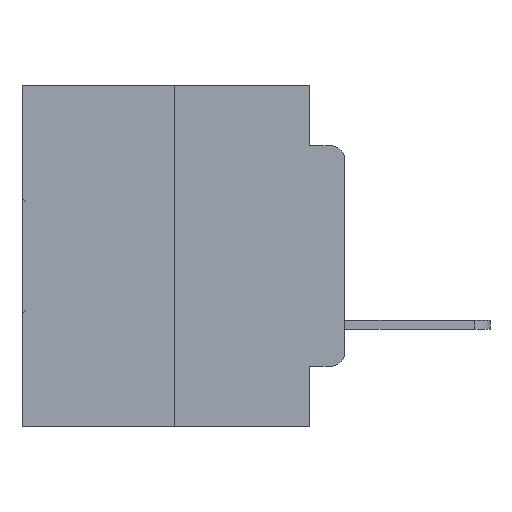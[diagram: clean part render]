
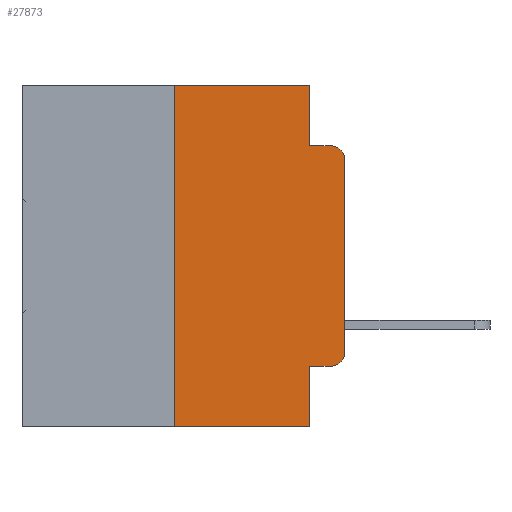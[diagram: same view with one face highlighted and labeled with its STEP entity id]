
A CAD part, left-side view. The second image highlights one B-rep face of the part: STEP entity #27873.
In plain terms, the highlighted planar face has unit normal (-1, 0, 0).
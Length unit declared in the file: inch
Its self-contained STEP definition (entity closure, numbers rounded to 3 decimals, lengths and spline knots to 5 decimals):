
#221 = EDGE_CURVE ( 'NONE', #346, #28090, #28840, .T. ) ;
#346 = VERTEX_POINT ( 'NONE', #8007 ) ;
#609 = LINE ( 'NONE', #29104, #14653 ) ;
#1253 = LINE ( 'NONE', #19078, #19991 ) ;
#1327 = EDGE_CURVE ( 'NONE', #11080, #346, #2122, .T. ) ;
#1549 = LINE ( 'NONE', #21572, #26983 ) ;
#1597 = VERTEX_POINT ( 'NONE', #19751 ) ;
#2122 = LINE ( 'NONE', #22585, #26089 ) ;
#2338 = CARTESIAN_POINT ( 'NONE',  ( 0., 0.02, -0.1085 ) ) ;
#3059 = ORIENTED_EDGE ( 'NONE', *, *, #221, .T. ) ;
#4509 = DIRECTION ( 'NONE',  ( 0., 0., -1. ) ) ;
#4846 = CARTESIAN_POINT ( 'NONE',  ( 0., 0.051, 0. ) ) ;
#5404 = CIRCLE ( 'NONE', #16463, 0.02 ) ;
#5990 = EDGE_CURVE ( 'NONE', #29400, #18457, #9635, .T. ) ;
#6635 = ORIENTED_EDGE ( 'NONE', *, *, #21454, .F. ) ;
#6990 = VERTEX_POINT ( 'NONE', #26063 ) ;
#7189 = DIRECTION ( 'NONE',  ( 0., 0., -1. ) ) ;
#7617 = LINE ( 'NONE', #24339, #30038 ) ;
#7746 = VERTEX_POINT ( 'NONE', #29175 ) ;
#7971 = DIRECTION ( 'NONE',  ( 0., -1., 0. ) ) ;
#7972 = CARTESIAN_POINT ( 'NONE',  ( 0., 0., -0.3915 ) ) ;
#8007 = CARTESIAN_POINT ( 'NONE',  ( 0., 0., -0.1085 ) ) ;
#8150 = EDGE_CURVE ( 'NONE', #6990, #7746, #1549, .T. ) ;
#8994 = VERTEX_POINT ( 'NONE', #11592 ) ;
#9467 = VERTEX_POINT ( 'NONE', #27816 ) ;
#9635 = LINE ( 'NONE', #15141, #26794 ) ;
#9763 = DIRECTION ( 'NONE',  ( 0., -1., 0. ) ) ;
#10082 = AXIS2_PLACEMENT_3D ( 'NONE', #27970, #18958, #4509 ) ;
#11080 = VERTEX_POINT ( 'NONE', #7972 ) ;
#11263 = ORIENTED_EDGE ( 'NONE', *, *, #1327, .T. ) ;
#11592 = CARTESIAN_POINT ( 'NONE',  ( 0., 0.051, -0.5 ) ) ;
#12137 = FACE_OUTER_BOUND ( 'NONE', #29045, .T. ) ;
#12693 = DIRECTION ( 'NONE',  ( 0., -1., 0. ) ) ;
#12794 = ORIENTED_EDGE ( 'NONE', *, *, #18736, .F. ) ;
#13134 = DIRECTION ( 'NONE',  ( 0., 0., -1. ) ) ;
#13972 = EDGE_CURVE ( 'NONE', #9467, #8994, #1253, .T. ) ;
#14167 = CARTESIAN_POINT ( 'NONE',  ( 0., 0.02, -0.3915 ) ) ;
#14268 = PLANE ( 'NONE',  #10082 ) ;
#14630 = EDGE_CURVE ( 'NONE', #1597, #28090, #7617, .T. ) ;
#14653 = VECTOR ( 'NONE', #13134, 39.37008 ) ;
#15141 = CARTESIAN_POINT ( 'NONE',  ( 0., 0.473, 0. ) ) ;
#15243 = LINE ( 'NONE', #19110, #20732 ) ;
#16463 = AXIS2_PLACEMENT_3D ( 'NONE', #14167, #30028, #16508 ) ;
#16508 = DIRECTION ( 'NONE',  ( 0., 0., -1. ) ) ;
#16810 = ORIENTED_EDGE ( 'NONE', *, *, #5990, .F. ) ;
#18341 = EDGE_CURVE ( 'NONE', #7746, #11080, #5404, .T. ) ;
#18457 = VERTEX_POINT ( 'NONE', #4846 ) ;
#18736 = EDGE_CURVE ( 'NONE', #18457, #1597, #15243, .T. ) ;
#18958 = DIRECTION ( 'NONE',  ( 1., 0., 0. ) ) ;
#19078 = CARTESIAN_POINT ( 'NONE',  ( 0., 0.473, -0.5 ) ) ;
#19110 = CARTESIAN_POINT ( 'NONE',  ( 0., 0.051, 0. ) ) ;
#19751 = CARTESIAN_POINT ( 'NONE',  ( 0., 0.051, -0.0885 ) ) ;
#19991 = VECTOR ( 'NONE', #25980, 39.37008 ) ;
#20496 = ORIENTED_EDGE ( 'NONE', *, *, #14630, .F. ) ;
#20588 = CARTESIAN_POINT ( 'NONE',  ( 0., 0.25, 0. ) ) ;
#20732 = VECTOR ( 'NONE', #7189, 39.37008 ) ;
#20906 = ORIENTED_EDGE ( 'NONE', *, *, #18341, .T. ) ;
#21226 = VECTOR ( 'NONE', #29564, 39.37008 ) ;
#21454 = EDGE_CURVE ( 'NONE', #6990, #8994, #609, .T. ) ;
#21572 = CARTESIAN_POINT ( 'NONE',  ( 0., 0.051, -0.4115 ) ) ;
#21602 = EDGE_CURVE ( 'NONE', #9467, #29400, #22720, .T. ) ;
#21955 = CARTESIAN_POINT ( 'NONE',  ( 0., 0.02, -0.0885 ) ) ;
#21999 = ORIENTED_EDGE ( 'NONE', *, *, #21602, .F. ) ;
#22585 = CARTESIAN_POINT ( 'NONE',  ( 0., 0., 0. ) ) ;
#22720 = LINE ( 'NONE', #20588, #21226 ) ;
#22728 = ORIENTED_EDGE ( 'NONE', *, *, #13972, .T. ) ;
#24339 = CARTESIAN_POINT ( 'NONE',  ( 0., 0.051, -0.0885 ) ) ;
#25421 = DIRECTION ( 'NONE',  ( 0., 0., 1. ) ) ;
#25980 = DIRECTION ( 'NONE',  ( 0., -1., 0. ) ) ;
#26063 = CARTESIAN_POINT ( 'NONE',  ( 0., 0.051, -0.4115 ) ) ;
#26089 = VECTOR ( 'NONE', #25421, 39.37008 ) ;
#26215 = DIRECTION ( 'NONE',  ( 0., 0., -1. ) ) ;
#26708 = CARTESIAN_POINT ( 'NONE',  ( 0., 0.25, 0. ) ) ;
#26794 = VECTOR ( 'NONE', #7971, 39.37008 ) ;
#26983 = VECTOR ( 'NONE', #9763, 39.37008 ) ;
#27816 = CARTESIAN_POINT ( 'NONE',  ( 0., 0.25, -0.5 ) ) ;
#27873 = ADVANCED_FACE ( 'NONE', ( #12137 ), #14268, .F. ) ;
#27970 = CARTESIAN_POINT ( 'NONE',  ( 0., 0.473, 0. ) ) ;
#28068 = AXIS2_PLACEMENT_3D ( 'NONE', #2338, #28210, #26215 ) ;
#28090 = VERTEX_POINT ( 'NONE', #21955 ) ;
#28210 = DIRECTION ( 'NONE',  ( -1., 0., 0. ) ) ;
#28610 = ORIENTED_EDGE ( 'NONE', *, *, #8150, .T. ) ;
#28840 = CIRCLE ( 'NONE', #28068, 0.02 ) ;
#29045 = EDGE_LOOP ( 'NONE', ( #11263, #3059, #20496, #12794, #16810, #21999, #22728, #6635, #28610, #20906 ) ) ;
#29104 = CARTESIAN_POINT ( 'NONE',  ( 0., 0.051, 0. ) ) ;
#29175 = CARTESIAN_POINT ( 'NONE',  ( 0., 0.02, -0.4115 ) ) ;
#29400 = VERTEX_POINT ( 'NONE', #26708 ) ;
#29564 = DIRECTION ( 'NONE',  ( 0., 0., 1. ) ) ;
#30028 = DIRECTION ( 'NONE',  ( -1., 0., 0. ) ) ;
#30038 = VECTOR ( 'NONE', #12693, 39.37008 ) ;
